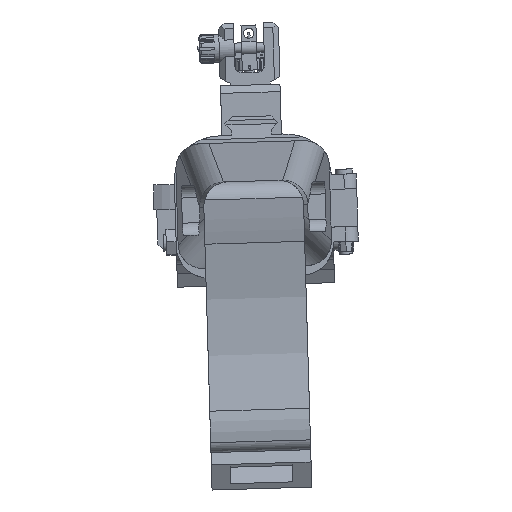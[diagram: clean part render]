
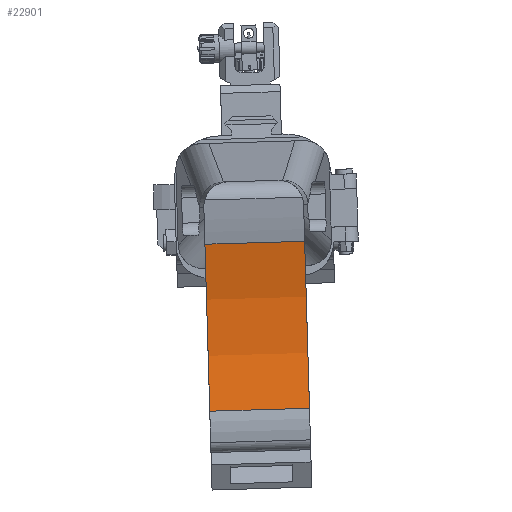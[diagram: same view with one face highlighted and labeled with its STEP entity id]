
A CAD part, left-side view. The second image highlights one B-rep face of the part: STEP entity #22901.
In plain terms, the highlighted cylindrical face has radius 137.628 mm (diameter 275.256 mm), a partial arc.
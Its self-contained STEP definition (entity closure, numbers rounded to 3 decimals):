
#329=CYLINDRICAL_SURFACE('',#24607,137.628);
#584=CIRCLE('',#24608,137.628);
#585=CIRCLE('',#24609,137.628);
#5195=ORIENTED_EDGE('',*,*,#9619,.T.);
#5196=ORIENTED_EDGE('',*,*,#9622,.T.);
#5197=ORIENTED_EDGE('',*,*,#9623,.F.);
#5198=ORIENTED_EDGE('',*,*,#9624,.F.);
#9619=EDGE_CURVE('',#12189,#12188,#14904,.T.);
#9622=EDGE_CURVE('',#12188,#12191,#584,.T.);
#9623=EDGE_CURVE('',#12192,#12191,#14905,.T.);
#9624=EDGE_CURVE('',#12189,#12192,#585,.T.);
#12188=VERTEX_POINT('',#35862);
#12189=VERTEX_POINT('',#35864);
#12191=VERTEX_POINT('',#35873);
#12192=VERTEX_POINT('',#35875);
#14904=LINE('',#35863,#17747);
#14905=LINE('',#35874,#17748);
#17747=VECTOR('',#29213,1000.);
#17748=VECTOR('',#29220,1000.);
#19393=EDGE_LOOP('',(#5195,#5196,#5197,#5198));
#20677=FACE_BOUND('',#19393,.T.);
#22901=ADVANCED_FACE('',(#20677),#329,.F.);
#24607=AXIS2_PLACEMENT_3D('',#35871,#29216,#29217);
#24608=AXIS2_PLACEMENT_3D('',#35872,#29218,#29219);
#24609=AXIS2_PLACEMENT_3D('',#35876,#29221,#29222);
#29213=DIRECTION('',(0.,1.,0.));
#29216=DIRECTION('',(0.,1.,0.));
#29217=DIRECTION('',(0.,0.,1.));
#29218=DIRECTION('',(0.,1.,0.));
#29219=DIRECTION('',(-1.,0.,0.));
#29220=DIRECTION('',(0.,1.,0.));
#29221=DIRECTION('',(0.,1.,0.));
#29222=DIRECTION('',(-1.,0.,0.));
#35862=CARTESIAN_POINT('',(-98.279,20.,67.356));
#35863=CARTESIAN_POINT('',(-98.279,-20.,67.356));
#35864=CARTESIAN_POINT('',(-98.279,-20.,67.356));
#35871=CARTESIAN_POINT('',(-231.77,-20.,33.869));
#35872=CARTESIAN_POINT('',(-231.77,20.,33.869));
#35873=CARTESIAN_POINT('',(-98.279,20.,0.382));
#35874=CARTESIAN_POINT('',(-98.279,-20.,0.382));
#35875=CARTESIAN_POINT('',(-98.279,-20.,0.382));
#35876=CARTESIAN_POINT('',(-231.77,-20.,33.869));
